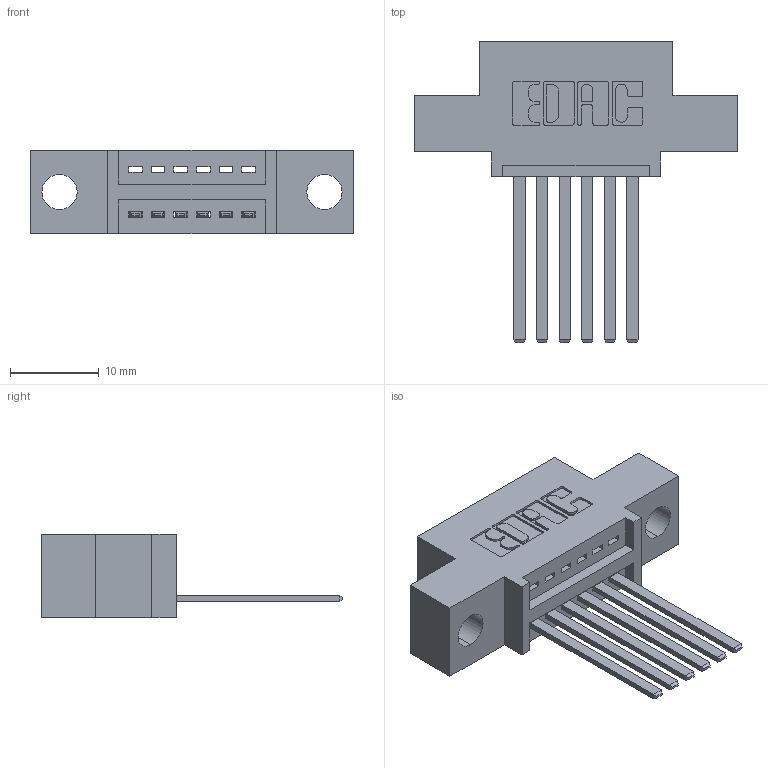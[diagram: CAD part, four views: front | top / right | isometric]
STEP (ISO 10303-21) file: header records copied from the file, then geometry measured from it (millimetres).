
FILE_DESCRIPTION (( 'STEP AP203' ), '1' );
FILE_NAME ('395-006-544-404.STEP', '2019-10-15T16:18:34', ( '' ), ( '' ), 'SwSTEP 2.0', 'SolidWorks 2016', '' );
FILE_SCHEMA (( 'CONFIG_CONTROL_DESIGN' ));
Length unit declared in the file: inch
Products named in the file (3): 345 Part_0.110 Offset - 0.156 Dia-TH; 395-006-544-404; 345-292-001_345-293-144
Assembly tree (7 placements, depth 2):
  395-006-544-404
    345 Part_0.110 Offset - 0.156 Dia-TH
    345-292-001_345-293-144  x6
Bounding box: 36.45 x 33.96 x 9.4 mm (x, y, z)
Volume: 3075.3 mm3; surface area: 3696.8 mm2
Topology: 7 solids, 7 shells, 442 faces, 1301 edges, 858 vertices
Faces by surface type: plane 300, cylinder 142
Entity records: 9313 total; most frequent: CARTESIAN_POINT 1622, ORIENTED_EDGE 1562, DIRECTION 1465, EDGE_CURVE 781, VECTOR 629, LINE 629, VERTEX_POINT 518, AXIS2_PLACEMENT_3D 418
